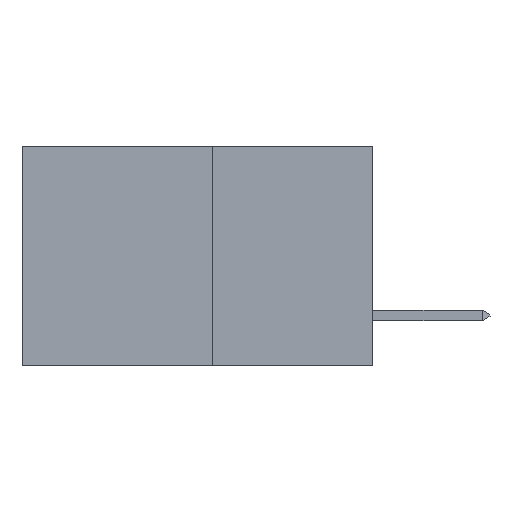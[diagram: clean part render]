
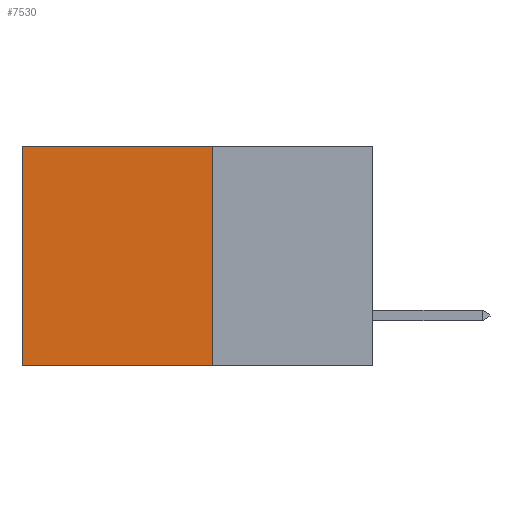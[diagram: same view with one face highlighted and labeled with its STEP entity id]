
A CAD part, left-side view. The second image highlights one B-rep face of the part: STEP entity #7530.
In plain terms, the highlighted planar face has unit normal (-1, 0, 0).
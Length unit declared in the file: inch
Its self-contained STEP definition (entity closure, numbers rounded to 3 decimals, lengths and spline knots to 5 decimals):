
#336 = FACE_OUTER_BOUND ( 'NONE', #2918, .T. ) ;
#1068 = DIRECTION ( 'NONE',  ( 0., 0., -1. ) ) ;
#1090 = CARTESIAN_POINT ( 'NONE',  ( 0.277, 0.59, -0.37 ) ) ;
#1256 = ORIENTED_EDGE ( 'NONE', *, *, #5011, .T. ) ;
#1378 = PLANE ( 'NONE',  #9296 ) ;
#2008 = VERTEX_POINT ( 'NONE', #6914 ) ;
#2079 = CARTESIAN_POINT ( 'NONE',  ( 0.277, 0.59, -0.37 ) ) ;
#2091 = VECTOR ( 'NONE', #7768, 39.37008 ) ;
#2587 = EDGE_CURVE ( 'NONE', #2008, #3861, #6058, .T. ) ;
#2918 = EDGE_LOOP ( 'NONE', ( #1256, #6534, #4792, #5111 ) ) ;
#2948 = LINE ( 'NONE', #9508, #5191 ) ;
#2989 = DIRECTION ( 'NONE',  ( 0., 1., 0. ) ) ;
#3472 = LINE ( 'NONE', #1090, #5217 ) ;
#3671 = CARTESIAN_POINT ( 'NONE',  ( 0.277, 0.27, -0.37 ) ) ;
#3694 = CARTESIAN_POINT ( 'NONE',  ( 0.277, 0.59, 0. ) ) ;
#3733 = DIRECTION ( 'NONE',  ( 1., 0., 0. ) ) ;
#3861 = VERTEX_POINT ( 'NONE', #3694 ) ;
#4300 = VERTEX_POINT ( 'NONE', #2079 ) ;
#4394 = VECTOR ( 'NONE', #7993, 39.37008 ) ;
#4792 = ORIENTED_EDGE ( 'NONE', *, *, #9218, .F. ) ;
#5011 = EDGE_CURVE ( 'NONE', #3861, #4300, #3472, .T. ) ;
#5111 = ORIENTED_EDGE ( 'NONE', *, *, #2587, .T. ) ;
#5191 = VECTOR ( 'NONE', #2989, 39.37008 ) ;
#5217 = VECTOR ( 'NONE', #1068, 39.37008 ) ;
#5795 = VERTEX_POINT ( 'NONE', #7554 ) ;
#6058 = LINE ( 'NONE', #8162, #2091 ) ;
#6072 = LINE ( 'NONE', #3671, #4394 ) ;
#6183 = EDGE_CURVE ( 'NONE', #5795, #4300, #2948, .T. ) ;
#6534 = ORIENTED_EDGE ( 'NONE', *, *, #6183, .F. ) ;
#6914 = CARTESIAN_POINT ( 'NONE',  ( 0.277, 0.27, 0. ) ) ;
#7530 = ADVANCED_FACE ( 'NONE', ( #336 ), #1378, .F. ) ;
#7554 = CARTESIAN_POINT ( 'NONE',  ( 0.277, 0.27, -0.37 ) ) ;
#7768 = DIRECTION ( 'NONE',  ( 0., 1., 0. ) ) ;
#7993 = DIRECTION ( 'NONE',  ( 0., 0., -1. ) ) ;
#8055 = CARTESIAN_POINT ( 'NONE',  ( 0.277, 0.27, -0.37 ) ) ;
#8162 = CARTESIAN_POINT ( 'NONE',  ( 0.277, 0.27, 0. ) ) ;
#8737 = DIRECTION ( 'NONE',  ( 0., 0., -1. ) ) ;
#9218 = EDGE_CURVE ( 'NONE', #2008, #5795, #6072, .T. ) ;
#9296 = AXIS2_PLACEMENT_3D ( 'NONE', #8055, #3733, #8737 ) ;
#9508 = CARTESIAN_POINT ( 'NONE',  ( 0.277, 0.27, -0.37 ) ) ;
